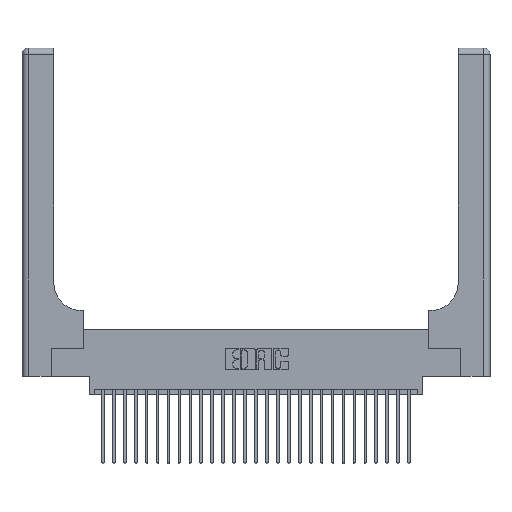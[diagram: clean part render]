
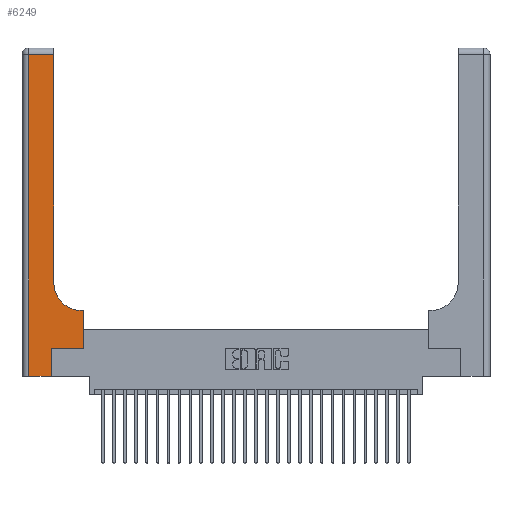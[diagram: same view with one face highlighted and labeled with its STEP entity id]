
A CAD part, top view. The second image highlights one B-rep face of the part: STEP entity #6249.
In plain terms, the highlighted planar face has unit normal (0, 0, 1).
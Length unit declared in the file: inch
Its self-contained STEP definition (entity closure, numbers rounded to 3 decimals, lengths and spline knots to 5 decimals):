
#318 = CARTESIAN_POINT ( 'NONE',  ( 0.06, 2.94, 0.37 ) ) ;
#423 = EDGE_CURVE ( 'NONE', #25134, #16160, #22535, .T. ) ;
#427 = VECTOR ( 'NONE', #8233, 39.37008 ) ;
#787 = CARTESIAN_POINT ( 'NONE',  ( 0.2915, 0.6, 0.37 ) ) ;
#1915 = VERTEX_POINT ( 'NONE', #17209 ) ;
#2477 = VECTOR ( 'NONE', #3187, 39.37008 ) ;
#2598 = ORIENTED_EDGE ( 'NONE', *, *, #13166, .T. ) ;
#3187 = DIRECTION ( 'NONE',  ( 0., 1., 0. ) ) ;
#3347 = LINE ( 'NONE', #5933, #25353 ) ;
#3925 = DIRECTION ( 'NONE',  ( 0., 1., 0. ) ) ;
#3937 = CARTESIAN_POINT ( 'NONE',  ( 0.5585, 0.25, 0.37 ) ) ;
#4281 = LINE ( 'NONE', #10234, #2477 ) ;
#4355 = DIRECTION ( 'NONE',  ( 0., 0., -1. ) ) ;
#4677 = VERTEX_POINT ( 'NONE', #12602 ) ;
#5597 = CARTESIAN_POINT ( 'NONE',  ( 0.5415, 0.85, 0.37 ) ) ;
#5626 = ORIENTED_EDGE ( 'NONE', *, *, #6111, .T. ) ;
#5933 = CARTESIAN_POINT ( 'NONE',  ( 0.269, 0., 0.37 ) ) ;
#6111 = EDGE_CURVE ( 'NONE', #18486, #4677, #13643, .T. ) ;
#6249 = ADVANCED_FACE ( 'NONE', ( #15127 ), #13695, .F. ) ;
#6331 = EDGE_CURVE ( 'NONE', #19248, #27620, #20570, .T. ) ;
#6563 = LINE ( 'NONE', #23449, #427 ) ;
#6769 = VECTOR ( 'NONE', #23355, 39.37008 ) ;
#7851 = LINE ( 'NONE', #23155, #6769 ) ;
#8233 = DIRECTION ( 'NONE',  ( -1., 0., 0. ) ) ;
#9468 = ORIENTED_EDGE ( 'NONE', *, *, #25237, .T. ) ;
#9666 = ORIENTED_EDGE ( 'NONE', *, *, #18751, .T. ) ;
#9830 = ORIENTED_EDGE ( 'NONE', *, *, #6331, .T. ) ;
#10218 = DIRECTION ( 'NONE',  ( 0., 0., -1. ) ) ;
#10234 = CARTESIAN_POINT ( 'NONE',  ( 0.2915, 3., 0.37 ) ) ;
#10244 = CARTESIAN_POINT ( 'NONE',  ( 0.5585, 0.6, 0.37 ) ) ;
#12602 = CARTESIAN_POINT ( 'NONE',  ( 0.06, 0., 0.37 ) ) ;
#13166 = EDGE_CURVE ( 'NONE', #24129, #18486, #6563, .T. ) ;
#13289 = LINE ( 'NONE', #787, #28058 ) ;
#13435 = DIRECTION ( 'NONE',  ( 0., -1., 0. ) ) ;
#13643 = LINE ( 'NONE', #15420, #24443 ) ;
#13695 = PLANE ( 'NONE',  #14535 ) ;
#14535 = AXIS2_PLACEMENT_3D ( 'NONE', #29855, #4355, #20457 ) ;
#15127 = FACE_OUTER_BOUND ( 'NONE', #22033, .T. ) ;
#15370 = ORIENTED_EDGE ( 'NONE', *, *, #29093, .T. ) ;
#15420 = CARTESIAN_POINT ( 'NONE',  ( 0.06, 3., 0.37 ) ) ;
#15497 = AXIS2_PLACEMENT_3D ( 'NONE', #5597, #10218, #19271 ) ;
#16160 = VERTEX_POINT ( 'NONE', #10244 ) ;
#16334 = CARTESIAN_POINT ( 'NONE',  ( 0., 0., 0.37 ) ) ;
#16794 = CARTESIAN_POINT ( 'NONE',  ( 0.2915, 0.85, 0.37 ) ) ;
#17209 = CARTESIAN_POINT ( 'NONE',  ( 0.269, 0., 0.37 ) ) ;
#17317 = VECTOR ( 'NONE', #26507, 39.37008 ) ;
#17705 = CARTESIAN_POINT ( 'NONE',  ( 0.2915, 2.94, 0.37 ) ) ;
#18178 = CARTESIAN_POINT ( 'NONE',  ( 0.5585, 0.25, 0.37 ) ) ;
#18486 = VERTEX_POINT ( 'NONE', #318 ) ;
#18751 = EDGE_CURVE ( 'NONE', #1915, #28269, #3347, .T. ) ;
#19248 = VERTEX_POINT ( 'NONE', #28687 ) ;
#19271 = DIRECTION ( 'NONE',  ( 1., 0., 0. ) ) ;
#19890 = CARTESIAN_POINT ( 'NONE',  ( 0.269, 0.25, 0.37 ) ) ;
#20176 = EDGE_CURVE ( 'NONE', #16160, #19248, #13289, .T. ) ;
#20253 = EDGE_CURVE ( 'NONE', #27620, #24129, #4281, .T. ) ;
#20457 = DIRECTION ( 'NONE',  ( -1., 0., 0. ) ) ;
#20570 = CIRCLE ( 'NONE', #15497, 0.25 ) ;
#21473 = DIRECTION ( 'NONE',  ( 0., 1., 0. ) ) ;
#22033 = EDGE_LOOP ( 'NONE', ( #26539, #2598, #5626, #9468, #9666, #15370, #29380, #27032, #9830 ) ) ;
#22535 = LINE ( 'NONE', #3937, #29782 ) ;
#23155 = CARTESIAN_POINT ( 'NONE',  ( 0.269, 0.25, 0.37 ) ) ;
#23355 = DIRECTION ( 'NONE',  ( 1., 0., 0. ) ) ;
#23449 = CARTESIAN_POINT ( 'NONE',  ( 0., 2.94, 0.37 ) ) ;
#23453 = LINE ( 'NONE', #16334, #17317 ) ;
#24129 = VERTEX_POINT ( 'NONE', #17705 ) ;
#24443 = VECTOR ( 'NONE', #13435, 39.37008 ) ;
#25134 = VERTEX_POINT ( 'NONE', #18178 ) ;
#25237 = EDGE_CURVE ( 'NONE', #4677, #1915, #23453, .T. ) ;
#25353 = VECTOR ( 'NONE', #3925, 39.37008 ) ;
#26507 = DIRECTION ( 'NONE',  ( 1., 0., 0. ) ) ;
#26539 = ORIENTED_EDGE ( 'NONE', *, *, #20253, .T. ) ;
#27032 = ORIENTED_EDGE ( 'NONE', *, *, #20176, .T. ) ;
#27620 = VERTEX_POINT ( 'NONE', #16794 ) ;
#28058 = VECTOR ( 'NONE', #28596, 39.37008 ) ;
#28269 = VERTEX_POINT ( 'NONE', #19890 ) ;
#28596 = DIRECTION ( 'NONE',  ( -1., 0., 0. ) ) ;
#28687 = CARTESIAN_POINT ( 'NONE',  ( 0.5415, 0.6, 0.37 ) ) ;
#29093 = EDGE_CURVE ( 'NONE', #28269, #25134, #7851, .T. ) ;
#29380 = ORIENTED_EDGE ( 'NONE', *, *, #423, .T. ) ;
#29782 = VECTOR ( 'NONE', #21473, 39.37008 ) ;
#29855 = CARTESIAN_POINT ( 'NONE',  ( 0., 3., 0.37 ) ) ;
